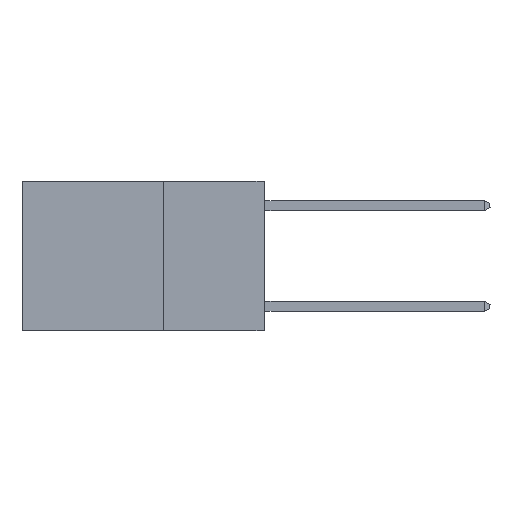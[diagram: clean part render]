
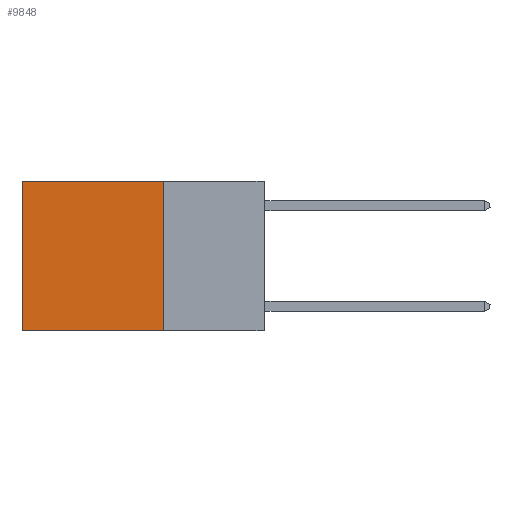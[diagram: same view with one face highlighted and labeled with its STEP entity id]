
A CAD part, left-side view. The second image highlights one B-rep face of the part: STEP entity #9848.
In plain terms, the highlighted planar face has unit normal (-1, 0, 0).
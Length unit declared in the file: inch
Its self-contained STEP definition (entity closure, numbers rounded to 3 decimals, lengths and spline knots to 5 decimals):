
#733 = LINE ( 'NONE', #16007, #11958 ) ;
#899 = DIRECTION ( 'NONE',  ( 0., 0., -1. ) ) ;
#2054 = AXIS2_PLACEMENT_3D ( 'NONE', #5900, #10077, #899 ) ;
#3743 = PLANE ( 'NONE',  #2054 ) ;
#4584 = DIRECTION ( 'NONE',  ( 0., 0., -1. ) ) ;
#4675 = LINE ( 'NONE', #12019, #10114 ) ;
#5353 = VECTOR ( 'NONE', #9379, 39.37008 ) ;
#5546 = VECTOR ( 'NONE', #7322, 39.37008 ) ;
#5793 = ORIENTED_EDGE ( 'NONE', *, *, #16338, .F. ) ;
#5900 = CARTESIAN_POINT ( 'NONE',  ( 0.2625, 0.25, 0. ) ) ;
#5983 = VERTEX_POINT ( 'NONE', #6252 ) ;
#6252 = CARTESIAN_POINT ( 'NONE',  ( 0.2625, 0.25, -0.37 ) ) ;
#6409 = ORIENTED_EDGE ( 'NONE', *, *, #11739, .T. ) ;
#6508 = CARTESIAN_POINT ( 'NONE',  ( 0.2625, 0.6, -0.37 ) ) ;
#6943 = CARTESIAN_POINT ( 'NONE',  ( 0.2625, 0.25, 0. ) ) ;
#7069 = VERTEX_POINT ( 'NONE', #6943 ) ;
#7322 = DIRECTION ( 'NONE',  ( 0., 1., 0. ) ) ;
#7598 = EDGE_CURVE ( 'NONE', #13450, #14094, #4675, .T. ) ;
#8167 = DIRECTION ( 'NONE',  ( 0., 0., -1. ) ) ;
#8571 = LINE ( 'NONE', #13680, #5546 ) ;
#9379 = DIRECTION ( 'NONE',  ( 0., 1., 0. ) ) ;
#9392 = EDGE_LOOP ( 'NONE', ( #9477, #5793, #10359, #6409 ) ) ;
#9477 = ORIENTED_EDGE ( 'NONE', *, *, #7598, .T. ) ;
#9614 = LINE ( 'NONE', #13408, #5353 ) ;
#9848 = ADVANCED_FACE ( 'NONE', ( #12515 ), #3743, .F. ) ;
#10077 = DIRECTION ( 'NONE',  ( 1., 0., 0. ) ) ;
#10114 = VECTOR ( 'NONE', #8167, 39.37008 ) ;
#10359 = ORIENTED_EDGE ( 'NONE', *, *, #12949, .F. ) ;
#10978 = CARTESIAN_POINT ( 'NONE',  ( 0.2625, 0.6, 0. ) ) ;
#11739 = EDGE_CURVE ( 'NONE', #7069, #13450, #8571, .T. ) ;
#11958 = VECTOR ( 'NONE', #4584, 39.37008 ) ;
#12019 = CARTESIAN_POINT ( 'NONE',  ( 0.2625, 0.6, 0. ) ) ;
#12515 = FACE_OUTER_BOUND ( 'NONE', #9392, .T. ) ;
#12949 = EDGE_CURVE ( 'NONE', #7069, #5983, #733, .T. ) ;
#13408 = CARTESIAN_POINT ( 'NONE',  ( 0.2625, 0.25, -0.37 ) ) ;
#13450 = VERTEX_POINT ( 'NONE', #10978 ) ;
#13680 = CARTESIAN_POINT ( 'NONE',  ( 0.2625, 0.25, 0. ) ) ;
#14094 = VERTEX_POINT ( 'NONE', #6508 ) ;
#16007 = CARTESIAN_POINT ( 'NONE',  ( 0.2625, 0.25, 0. ) ) ;
#16338 = EDGE_CURVE ( 'NONE', #5983, #14094, #9614, .T. ) ;
